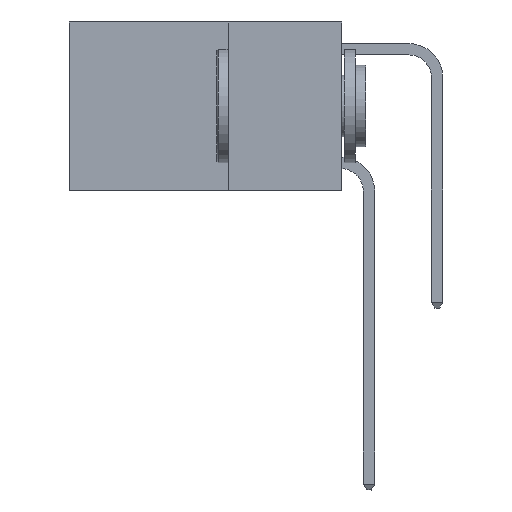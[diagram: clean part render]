
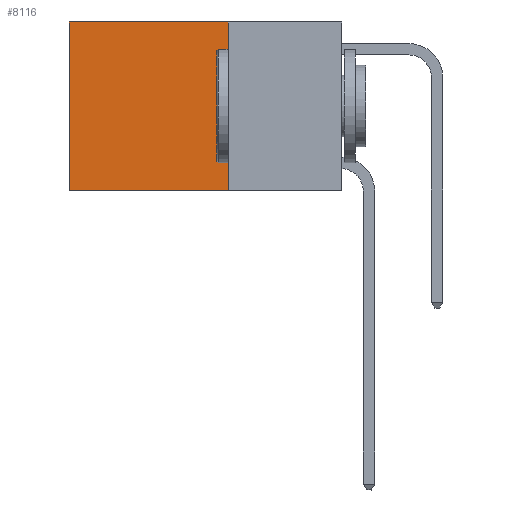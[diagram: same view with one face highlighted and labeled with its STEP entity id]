
A CAD part, left-side view. The second image highlights one B-rep face of the part: STEP entity #8116.
In plain terms, the highlighted planar face has unit normal (-1, 0, 0).
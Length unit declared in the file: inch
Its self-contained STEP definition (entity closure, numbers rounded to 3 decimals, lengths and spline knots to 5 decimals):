
#32 = AXIS2_PLACEMENT_3D ( 'NONE', #3589, #8767, #3629 ) ;
#1200 = ORIENTED_EDGE ( 'NONE', *, *, #5670, .T. ) ;
#1289 = DIRECTION ( 'NONE',  ( 0., 0., -1. ) ) ;
#2048 = ORIENTED_EDGE ( 'NONE', *, *, #9620, .T. ) ;
#2378 = EDGE_CURVE ( 'NONE', #4806, #6581, #9222, .T. ) ;
#2418 = ORIENTED_EDGE ( 'NONE', *, *, #3253, .F. ) ;
#3037 = ORIENTED_EDGE ( 'NONE', *, *, #2378, .F. ) ;
#3060 = CARTESIAN_POINT ( 'NONE',  ( 0.2625, 0.25, 0. ) ) ;
#3253 = EDGE_CURVE ( 'NONE', #8478, #4806, #6725, .T. ) ;
#3513 = DIRECTION ( 'NONE',  ( 0., 0., -1. ) ) ;
#3537 = CARTESIAN_POINT ( 'NONE',  ( 0.2625, 0.6, -0.37 ) ) ;
#3589 = CARTESIAN_POINT ( 'NONE',  ( 0.2625, 0.25, 0. ) ) ;
#3629 = DIRECTION ( 'NONE',  ( 0., 0., -1. ) ) ;
#3883 = EDGE_LOOP ( 'NONE', ( #1200, #3037, #2418, #2048 ) ) ;
#4192 = DIRECTION ( 'NONE',  ( 0., 1., 0. ) ) ;
#4267 = FACE_OUTER_BOUND ( 'NONE', #3883, .T. ) ;
#4486 = VECTOR ( 'NONE', #3513, 39.37008 ) ;
#4520 = VECTOR ( 'NONE', #1289, 39.37008 ) ;
#4806 = VERTEX_POINT ( 'NONE', #6823 ) ;
#5072 = CARTESIAN_POINT ( 'NONE',  ( 0.2625, 0.25, 0. ) ) ;
#5188 = CARTESIAN_POINT ( 'NONE',  ( 0.2625, 0.6, 0. ) ) ;
#5670 = EDGE_CURVE ( 'NONE', #9744, #6581, #7466, .T. ) ;
#6138 = PLANE ( 'NONE',  #32 ) ;
#6581 = VERTEX_POINT ( 'NONE', #3537 ) ;
#6725 = LINE ( 'NONE', #3060, #4520 ) ;
#6823 = CARTESIAN_POINT ( 'NONE',  ( 0.2625, 0.25, -0.37 ) ) ;
#7118 = LINE ( 'NONE', #9216, #9174 ) ;
#7466 = LINE ( 'NONE', #5188, #4486 ) ;
#8116 = ADVANCED_FACE ( 'NONE', ( #4267 ), #6138, .F. ) ;
#8478 = VERTEX_POINT ( 'NONE', #5072 ) ;
#8767 = DIRECTION ( 'NONE',  ( 1., 0., 0. ) ) ;
#8960 = VECTOR ( 'NONE', #4192, 39.37008 ) ;
#9174 = VECTOR ( 'NONE', #10040, 39.37008 ) ;
#9216 = CARTESIAN_POINT ( 'NONE',  ( 0.2625, 0.25, 0. ) ) ;
#9222 = LINE ( 'NONE', #9309, #8960 ) ;
#9309 = CARTESIAN_POINT ( 'NONE',  ( 0.2625, 0.25, -0.37 ) ) ;
#9327 = CARTESIAN_POINT ( 'NONE',  ( 0.2625, 0.6, 0. ) ) ;
#9620 = EDGE_CURVE ( 'NONE', #8478, #9744, #7118, .T. ) ;
#9744 = VERTEX_POINT ( 'NONE', #9327 ) ;
#10040 = DIRECTION ( 'NONE',  ( 0., 1., 0. ) ) ;
